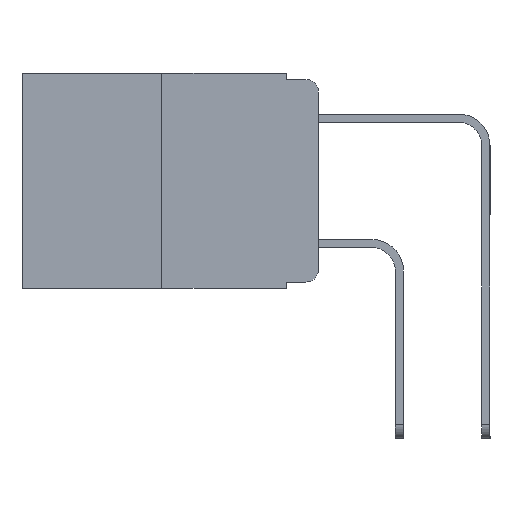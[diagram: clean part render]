
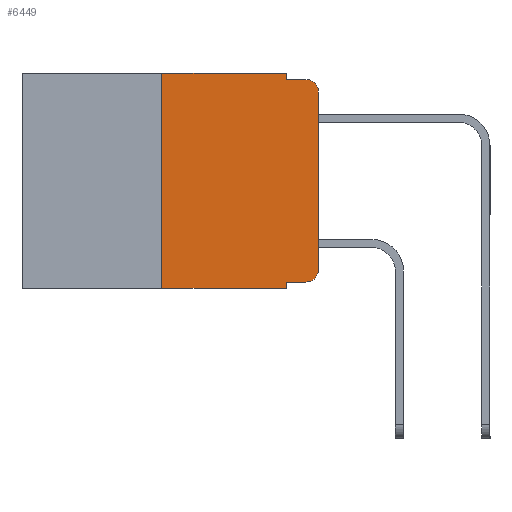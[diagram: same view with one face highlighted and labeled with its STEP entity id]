
A CAD part, left-side view. The second image highlights one B-rep face of the part: STEP entity #6449.
In plain terms, the highlighted planar face has unit normal (-1, 0, 0).
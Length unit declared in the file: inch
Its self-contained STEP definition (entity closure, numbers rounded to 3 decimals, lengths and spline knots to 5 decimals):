
#47 = ORIENTED_EDGE ( 'NONE', *, *, #296, .T. ) ;
#296 = EDGE_CURVE ( 'NONE', #13780, #8486, #15823, .T. ) ;
#480 = CARTESIAN_POINT ( 'NONE',  ( 0., 0.051, -0.01 ) ) ;
#817 = CARTESIAN_POINT ( 'NONE',  ( 0., 0.25, -0.343 ) ) ;
#1453 = DIRECTION ( 'NONE',  ( 0., 0., -1. ) ) ;
#1550 = EDGE_CURVE ( 'NONE', #13780, #16472, #7656, .T. ) ;
#1780 = VERTEX_POINT ( 'NONE', #20707 ) ;
#2166 = EDGE_LOOP ( 'NONE', ( #10684, #9927, #8672, #3295, #6444, #12138, #12217, #12402, #47, #6400 ) ) ;
#2337 = AXIS2_PLACEMENT_3D ( 'NONE', #9556, #16494, #6136 ) ;
#2363 = DIRECTION ( 'NONE',  ( 0., -1., 0. ) ) ;
#2584 = CARTESIAN_POINT ( 'NONE',  ( 0., 0.02, -0.333 ) ) ;
#2798 = EDGE_CURVE ( 'NONE', #6498, #10642, #3322, .T. ) ;
#2801 = DIRECTION ( 'NONE',  ( 0., 0., -1. ) ) ;
#2952 = VECTOR ( 'NONE', #6299, 39.37008 ) ;
#3295 = ORIENTED_EDGE ( 'NONE', *, *, #3972, .F. ) ;
#3322 = LINE ( 'NONE', #12080, #7487 ) ;
#3695 = CARTESIAN_POINT ( 'NONE',  ( 0., 0.051, -0.343 ) ) ;
#3972 = EDGE_CURVE ( 'NONE', #18920, #1780, #6060, .T. ) ;
#4073 = VERTEX_POINT ( 'NONE', #15328 ) ;
#4321 = PLANE ( 'NONE',  #2337 ) ;
#4664 = DIRECTION ( 'NONE',  ( 0., 0., 1. ) ) ;
#4902 = CARTESIAN_POINT ( 'NONE',  ( 0., 0.02, -0.01 ) ) ;
#5569 = LINE ( 'NONE', #15857, #18862 ) ;
#5955 = FACE_OUTER_BOUND ( 'NONE', #2166, .T. ) ;
#6060 = LINE ( 'NONE', #15026, #19354 ) ;
#6136 = DIRECTION ( 'NONE',  ( 0., 0., -1. ) ) ;
#6219 = CARTESIAN_POINT ( 'NONE',  ( 0., 0.051, 0. ) ) ;
#6244 = DIRECTION ( 'NONE',  ( 0., 0., 1. ) ) ;
#6299 = DIRECTION ( 'NONE',  ( 0., 0., -1. ) ) ;
#6381 = EDGE_CURVE ( 'NONE', #1780, #21489, #11089, .T. ) ;
#6400 = ORIENTED_EDGE ( 'NONE', *, *, #21624, .T. ) ;
#6444 = ORIENTED_EDGE ( 'NONE', *, *, #12027, .F. ) ;
#6449 = ADVANCED_FACE ( 'NONE', ( #5955 ), #4321, .F. ) ;
#6498 = VERTEX_POINT ( 'NONE', #817 ) ;
#6904 = CARTESIAN_POINT ( 'NONE',  ( 0., 0.051, 0. ) ) ;
#7052 = VECTOR ( 'NONE', #2363, 39.37008 ) ;
#7487 = VECTOR ( 'NONE', #4664, 39.37008 ) ;
#7656 = LINE ( 'NONE', #6904, #2952 ) ;
#7930 = AXIS2_PLACEMENT_3D ( 'NONE', #10490, #22570, #12184 ) ;
#8486 = VERTEX_POINT ( 'NONE', #2584 ) ;
#8672 = ORIENTED_EDGE ( 'NONE', *, *, #6381, .F. ) ;
#8719 = EDGE_CURVE ( 'NONE', #21404, #21489, #9689, .T. ) ;
#9556 = CARTESIAN_POINT ( 'NONE',  ( 0., 0.473, 0. ) ) ;
#9689 = CIRCLE ( 'NONE', #17279, 0.02 ) ;
#9927 = ORIENTED_EDGE ( 'NONE', *, *, #8719, .T. ) ;
#10490 = CARTESIAN_POINT ( 'NONE',  ( 0., 0.02, -0.313 ) ) ;
#10642 = VERTEX_POINT ( 'NONE', #16169 ) ;
#10684 = ORIENTED_EDGE ( 'NONE', *, *, #11012, .T. ) ;
#11012 = EDGE_CURVE ( 'NONE', #4073, #21404, #22167, .T. ) ;
#11089 = LINE ( 'NONE', #480, #7052 ) ;
#11986 = DIRECTION ( 'NONE',  ( -1., 0., 0. ) ) ;
#12027 = EDGE_CURVE ( 'NONE', #10642, #18920, #5569, .T. ) ;
#12080 = CARTESIAN_POINT ( 'NONE',  ( 0., 0.25, 0. ) ) ;
#12138 = ORIENTED_EDGE ( 'NONE', *, *, #2798, .F. ) ;
#12184 = DIRECTION ( 'NONE',  ( 0., 0., -1. ) ) ;
#12217 = ORIENTED_EDGE ( 'NONE', *, *, #16368, .T. ) ;
#12402 = ORIENTED_EDGE ( 'NONE', *, *, #1550, .F. ) ;
#13780 = VERTEX_POINT ( 'NONE', #17967 ) ;
#14191 = DIRECTION ( 'NONE',  ( 0., -1., 0. ) ) ;
#14525 = CARTESIAN_POINT ( 'NONE',  ( 0., 0.051, -0.333 ) ) ;
#14658 = VECTOR ( 'NONE', #17383, 39.37008 ) ;
#14755 = VECTOR ( 'NONE', #14191, 39.37008 ) ;
#15026 = CARTESIAN_POINT ( 'NONE',  ( 0., 0.051, 0. ) ) ;
#15218 = LINE ( 'NONE', #22564, #14658 ) ;
#15328 = CARTESIAN_POINT ( 'NONE',  ( 0., 0., -0.313 ) ) ;
#15823 = LINE ( 'NONE', #14525, #14755 ) ;
#15857 = CARTESIAN_POINT ( 'NONE',  ( 0., 0.473, 0. ) ) ;
#16169 = CARTESIAN_POINT ( 'NONE',  ( 0., 0.25, 0. ) ) ;
#16368 = EDGE_CURVE ( 'NONE', #6498, #16472, #15218, .T. ) ;
#16472 = VERTEX_POINT ( 'NONE', #3695 ) ;
#16494 = DIRECTION ( 'NONE',  ( 1., 0., 0. ) ) ;
#17004 = VECTOR ( 'NONE', #6244, 39.37008 ) ;
#17279 = AXIS2_PLACEMENT_3D ( 'NONE', #22384, #11986, #1453 ) ;
#17383 = DIRECTION ( 'NONE',  ( 0., -1., 0. ) ) ;
#17590 = DIRECTION ( 'NONE',  ( 0., -1., 0. ) ) ;
#17967 = CARTESIAN_POINT ( 'NONE',  ( 0., 0.051, -0.333 ) ) ;
#18232 = CARTESIAN_POINT ( 'NONE',  ( 0., 0., 0. ) ) ;
#18477 = CARTESIAN_POINT ( 'NONE',  ( 0., 0., -0.03 ) ) ;
#18862 = VECTOR ( 'NONE', #17590, 39.37008 ) ;
#18920 = VERTEX_POINT ( 'NONE', #6219 ) ;
#19354 = VECTOR ( 'NONE', #2801, 39.37008 ) ;
#20707 = CARTESIAN_POINT ( 'NONE',  ( 0., 0.051, -0.01 ) ) ;
#20711 = CIRCLE ( 'NONE', #7930, 0.02 ) ;
#21404 = VERTEX_POINT ( 'NONE', #18477 ) ;
#21489 = VERTEX_POINT ( 'NONE', #4902 ) ;
#21624 = EDGE_CURVE ( 'NONE', #8486, #4073, #20711, .T. ) ;
#22167 = LINE ( 'NONE', #18232, #17004 ) ;
#22384 = CARTESIAN_POINT ( 'NONE',  ( 0., 0.02, -0.03 ) ) ;
#22564 = CARTESIAN_POINT ( 'NONE',  ( 0., 0.473, -0.343 ) ) ;
#22570 = DIRECTION ( 'NONE',  ( -1., 0., 0. ) ) ;
